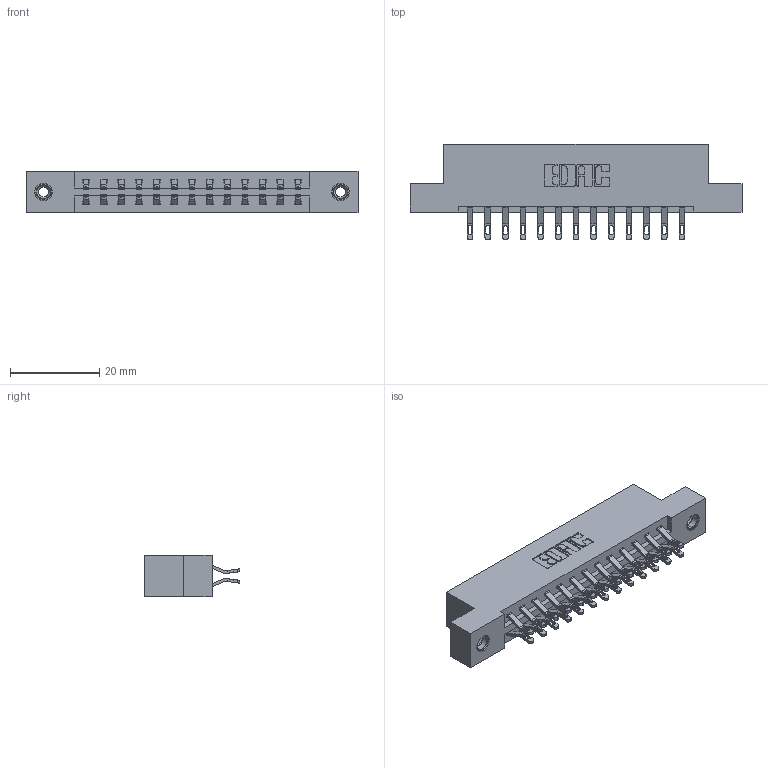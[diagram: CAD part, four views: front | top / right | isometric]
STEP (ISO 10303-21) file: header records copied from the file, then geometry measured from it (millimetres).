
FILE_DESCRIPTION (( 'STEP AP203' ), '1' );
FILE_NAME ('387-026-555-208.STEP', '2019-10-16T20:33:13', ( '' ), ( '' ), 'SwSTEP 2.0', 'SolidWorks 2016', '' );
FILE_SCHEMA (( 'CONFIG_CONTROL_DESIGN' ));
Length unit declared in the file: inch
Products named in the file (4): 337 Part_Flush Mounting Lugs - 0.156 Dia-TI; 345-250-001_345-250-003-102; 345-292-001_555 Tail; 387-026-555-208
Assembly tree (29 placements, depth 2):
  387-026-555-208
    337 Part_Flush Mounting Lugs - 0.156 Dia-TI
    345-292-001_555 Tail  x26
    345-250-001_345-250-003-102  x2
Bounding box: 74.52 x 21.47 x 9.4 mm (x, y, z)
Volume: 7536.8 mm3; surface area: 8546.8 mm2
Topology: 29 solids, 29 shells, 1734 faces, 5361 edges, 3566 vertices
Faces by surface type: plane 1038, cylinder 680, cone 12, torus 4
Entity records: 15342 total; most frequent: CARTESIAN_POINT 2623, ORIENTED_EDGE 2522, DIRECTION 2287, EDGE_CURVE 1261, LINE 1093, VECTOR 1093, VERTEX_POINT 836, AXIS2_PLACEMENT_3D 597
